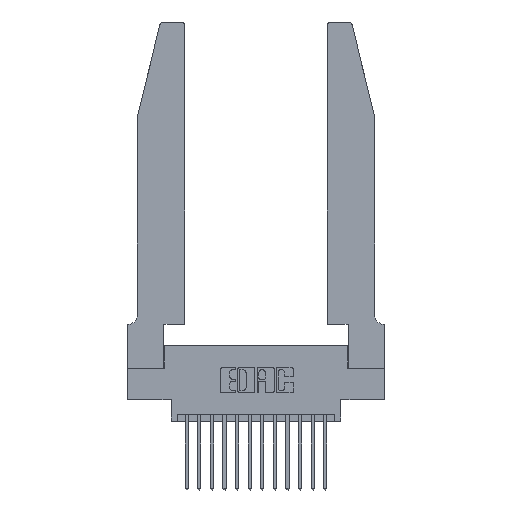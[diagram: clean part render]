
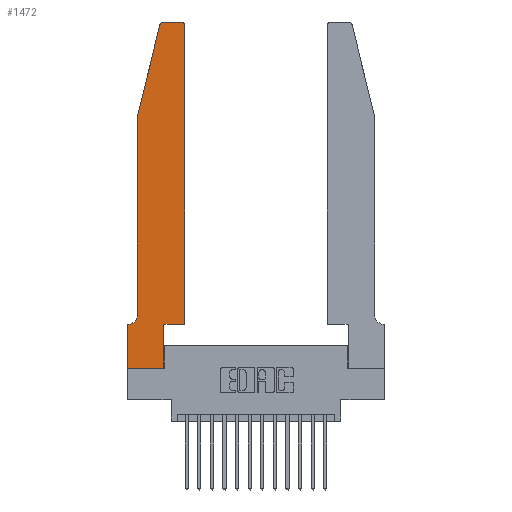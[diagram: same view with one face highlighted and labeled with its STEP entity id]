
A CAD part, top view. The second image highlights one B-rep face of the part: STEP entity #1472.
In plain terms, the highlighted planar face has unit normal (0, 0, 1).
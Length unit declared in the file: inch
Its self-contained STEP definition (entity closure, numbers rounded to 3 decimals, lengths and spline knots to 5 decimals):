
#182 = CARTESIAN_POINT ( 'NONE',  ( 0.4205, 2.72, 0.37 ) ) ;
#254 = CARTESIAN_POINT ( 'NONE',  ( 0.284, 2.72, 0.37 ) ) ;
#563 = ORIENTED_EDGE ( 'NONE', *, *, #5249, .T. ) ;
#570 = LINE ( 'NONE', #17295, #3205 ) ;
#616 = ORIENTED_EDGE ( 'NONE', *, *, #12248, .T. ) ;
#725 = CARTESIAN_POINT ( 'NONE',  ( 0.4505, 2.72, 0.37 ) ) ;
#1221 = EDGE_CURVE ( 'NONE', #15432, #1336, #11500, .T. ) ;
#1294 = VECTOR ( 'NONE', #11275, 39.37008 ) ;
#1336 = VERTEX_POINT ( 'NONE', #725 ) ;
#1472 = ADVANCED_FACE ( 'NONE', ( #15513 ), #16753, .T. ) ;
#1554 = EDGE_CURVE ( 'NONE', #3783, #7199, #5059, .T. ) ;
#1961 = ORIENTED_EDGE ( 'NONE', *, *, #5147, .T. ) ;
#2055 = CARTESIAN_POINT ( 'NONE',  ( 0.0755, 2., 0.37 ) ) ;
#2385 = DIRECTION ( 'NONE',  ( 0., 0., 1. ) ) ;
#2490 = EDGE_CURVE ( 'NONE', #15866, #15432, #9458, .T. ) ;
#2513 = ORIENTED_EDGE ( 'NONE', *, *, #5731, .T. ) ;
#2688 = CARTESIAN_POINT ( 'NONE',  ( 0., 0., 0.37 ) ) ;
#3089 = DIRECTION ( 'NONE',  ( -1., 0., 0. ) ) ;
#3205 = VECTOR ( 'NONE', #3089, 39.37008 ) ;
#3310 = DIRECTION ( 'NONE',  ( 0., 1., 0. ) ) ;
#3329 = CARTESIAN_POINT ( 'NONE',  ( 0.25487, 2.72718, 0.37 ) ) ;
#3634 = ORIENTED_EDGE ( 'NONE', *, *, #17968, .T. ) ;
#3783 = VERTEX_POINT ( 'NONE', #16994 ) ;
#3841 = VECTOR ( 'NONE', #6215, 39.37008 ) ;
#3972 = VECTOR ( 'NONE', #3310, 39.37008 ) ;
#4325 = DIRECTION ( 'NONE',  ( 0., 0., 1. ) ) ;
#4402 = CARTESIAN_POINT ( 'NONE',  ( 0.0055, 0.35, 0.37 ) ) ;
#4993 = CARTESIAN_POINT ( 'NONE',  ( 0.0755, 2., 0.37 ) ) ;
#5059 = LINE ( 'NONE', #18361, #1294 ) ;
#5147 = EDGE_CURVE ( 'NONE', #10669, #14370, #6265, .T. ) ;
#5249 = EDGE_CURVE ( 'NONE', #7199, #8905, #13153, .T. ) ;
#5363 = CIRCLE ( 'NONE', #17681, 0.03 ) ;
#5731 = EDGE_CURVE ( 'NONE', #16868, #15804, #11991, .T. ) ;
#6208 = CARTESIAN_POINT ( 'NONE',  ( 0.4505, 0.35, 0.37 ) ) ;
#6215 = DIRECTION ( 'NONE',  ( -0.239, -0.971, 0. ) ) ;
#6265 = LINE ( 'NONE', #4993, #3841 ) ;
#7199 = VERTEX_POINT ( 'NONE', #13962 ) ;
#7443 = DIRECTION ( 'NONE',  ( 1., 0., 0. ) ) ;
#7527 = CARTESIAN_POINT ( 'NONE',  ( 0.0755, 0.35, 0.37 ) ) ;
#7876 = CARTESIAN_POINT ( 'NONE',  ( 0.284, 2.75, 0.37 ) ) ;
#8297 = ORIENTED_EDGE ( 'NONE', *, *, #1554, .T. ) ;
#8384 = ORIENTED_EDGE ( 'NONE', *, *, #16856, .T. ) ;
#8697 = LINE ( 'NONE', #17689, #9781 ) ;
#8905 = VERTEX_POINT ( 'NONE', #11386 ) ;
#8981 = VECTOR ( 'NONE', #18282, 39.37008 ) ;
#9245 = EDGE_LOOP ( 'NONE', ( #16883, #15899, #1961, #17171, #2513, #8384, #8297, #563, #616, #13704, #17813, #3634 ) ) ;
#9458 = LINE ( 'NONE', #17164, #16367 ) ;
#9781 = VECTOR ( 'NONE', #18164, 39.37008 ) ;
#10065 = CIRCLE ( 'NONE', #16331, 0.03 ) ;
#10146 = DIRECTION ( 'NONE',  ( 0., 0., 1. ) ) ;
#10451 = CARTESIAN_POINT ( 'NONE',  ( 0.0055, 0.42, 0.37 ) ) ;
#10515 = LINE ( 'NONE', #16809, #8981 ) ;
#10540 = EDGE_CURVE ( 'NONE', #12307, #12216, #570, .T. ) ;
#10669 = VERTEX_POINT ( 'NONE', #3329 ) ;
#11030 = CARTESIAN_POINT ( 'NONE',  ( 0., 0.35, 0.37 ) ) ;
#11275 = DIRECTION ( 'NONE',  ( 0., -1., 0. ) ) ;
#11386 = CARTESIAN_POINT ( 'NONE',  ( 0.2865, 0., 0.37 ) ) ;
#11500 = LINE ( 'NONE', #13155, #3972 ) ;
#11705 = AXIS2_PLACEMENT_3D ( 'NONE', #11030, #2385, #13725 ) ;
#11991 = CIRCLE ( 'NONE', #17596, 0.07 ) ;
#12137 = EDGE_CURVE ( 'NONE', #12216, #10669, #5363, .T. ) ;
#12216 = VERTEX_POINT ( 'NONE', #7876 ) ;
#12248 = EDGE_CURVE ( 'NONE', #8905, #15866, #8697, .T. ) ;
#12307 = VERTEX_POINT ( 'NONE', #12438 ) ;
#12438 = CARTESIAN_POINT ( 'NONE',  ( 0.4205, 2.75, 0.37 ) ) ;
#12767 = CARTESIAN_POINT ( 'NONE',  ( 0.2865, 0.35, 0.37 ) ) ;
#13153 = LINE ( 'NONE', #2688, #17605 ) ;
#13155 = CARTESIAN_POINT ( 'NONE',  ( 0.4505, 0.35, 0.37 ) ) ;
#13610 = CARTESIAN_POINT ( 'NONE',  ( 0.0755, 0.42, 0.37 ) ) ;
#13704 = ORIENTED_EDGE ( 'NONE', *, *, #2490, .T. ) ;
#13725 = DIRECTION ( 'NONE',  ( 1., 0., 0. ) ) ;
#13962 = CARTESIAN_POINT ( 'NONE',  ( 0., 0., 0.37 ) ) ;
#14370 = VERTEX_POINT ( 'NONE', #2055 ) ;
#14391 = DIRECTION ( 'NONE',  ( 1., 0., 0. ) ) ;
#15432 = VERTEX_POINT ( 'NONE', #6208 ) ;
#15453 = VECTOR ( 'NONE', #17471, 39.37008 ) ;
#15513 = FACE_OUTER_BOUND ( 'NONE', #9245, .T. ) ;
#15804 = VERTEX_POINT ( 'NONE', #4402 ) ;
#15866 = VERTEX_POINT ( 'NONE', #12767 ) ;
#15899 = ORIENTED_EDGE ( 'NONE', *, *, #12137, .T. ) ;
#16331 = AXIS2_PLACEMENT_3D ( 'NONE', #182, #4325, #14391 ) ;
#16367 = VECTOR ( 'NONE', #18386, 39.37008 ) ;
#16621 = DIRECTION ( 'NONE',  ( 0., 0., -1. ) ) ;
#16753 = PLANE ( 'NONE',  #11705 ) ;
#16809 = CARTESIAN_POINT ( 'NONE',  ( 0.0755, 2., 0.37 ) ) ;
#16856 = EDGE_CURVE ( 'NONE', #15804, #3783, #17433, .T. ) ;
#16868 = VERTEX_POINT ( 'NONE', #13610 ) ;
#16883 = ORIENTED_EDGE ( 'NONE', *, *, #10540, .T. ) ;
#16956 = DIRECTION ( 'NONE',  ( 1., 0., 0. ) ) ;
#16994 = CARTESIAN_POINT ( 'NONE',  ( 0., 0.35, 0.37 ) ) ;
#17164 = CARTESIAN_POINT ( 'NONE',  ( 0.4505, 0.35, 0.37 ) ) ;
#17171 = ORIENTED_EDGE ( 'NONE', *, *, #17844, .T. ) ;
#17295 = CARTESIAN_POINT ( 'NONE',  ( 0.2605, 2.75, 0.37 ) ) ;
#17433 = LINE ( 'NONE', #7527, #15453 ) ;
#17471 = DIRECTION ( 'NONE',  ( -1., 0., 0. ) ) ;
#17495 = DIRECTION ( 'NONE',  ( -1., 0., 0. ) ) ;
#17596 = AXIS2_PLACEMENT_3D ( 'NONE', #10451, #16621, #17495 ) ;
#17605 = VECTOR ( 'NONE', #16956, 39.37008 ) ;
#17681 = AXIS2_PLACEMENT_3D ( 'NONE', #254, #10146, #7443 ) ;
#17689 = CARTESIAN_POINT ( 'NONE',  ( 0.2865, 0.35, 0.37 ) ) ;
#17813 = ORIENTED_EDGE ( 'NONE', *, *, #1221, .T. ) ;
#17844 = EDGE_CURVE ( 'NONE', #14370, #16868, #10515, .T. ) ;
#17968 = EDGE_CURVE ( 'NONE', #1336, #12307, #10065, .T. ) ;
#18164 = DIRECTION ( 'NONE',  ( 0., 1., 0. ) ) ;
#18282 = DIRECTION ( 'NONE',  ( 0., -1., 0. ) ) ;
#18361 = CARTESIAN_POINT ( 'NONE',  ( 0., 0., 0.37 ) ) ;
#18386 = DIRECTION ( 'NONE',  ( 1., 0., 0. ) ) ;
